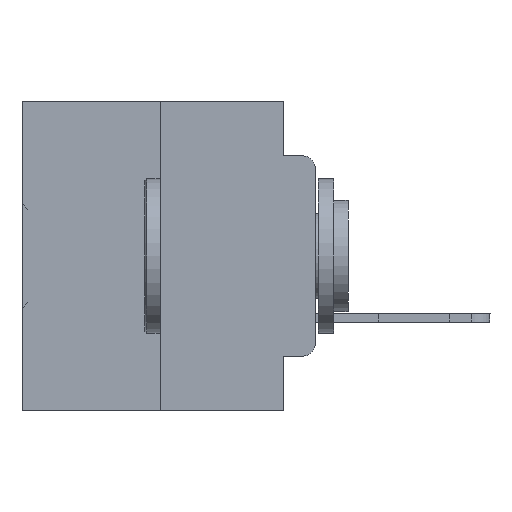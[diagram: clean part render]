
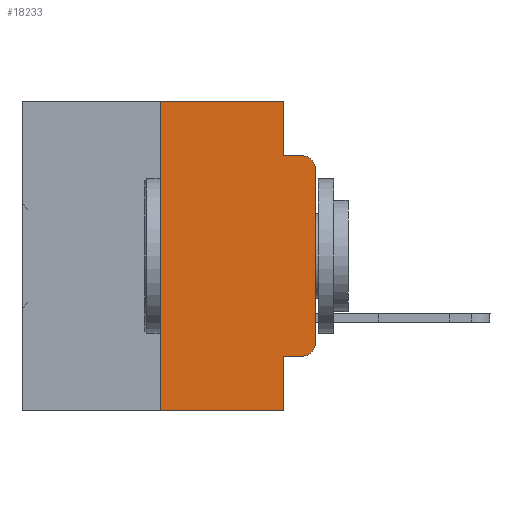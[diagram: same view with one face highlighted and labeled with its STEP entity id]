
A CAD part, left-side view. The second image highlights one B-rep face of the part: STEP entity #18233.
In plain terms, the highlighted planar face has unit normal (-1, 0, 0).
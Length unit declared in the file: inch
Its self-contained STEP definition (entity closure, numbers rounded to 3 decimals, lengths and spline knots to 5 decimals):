
#731 = VECTOR ( 'NONE', #1885, 39.37008 ) ;
#1237 = ORIENTED_EDGE ( 'NONE', *, *, #8486, .T. ) ;
#1719 = ORIENTED_EDGE ( 'NONE', *, *, #9011, .F. ) ;
#1763 = LINE ( 'NONE', #30060, #22072 ) ;
#1885 = DIRECTION ( 'NONE',  ( 0., 0., 1. ) ) ;
#2205 = CARTESIAN_POINT ( 'NONE',  ( 0., 0.051, -0.0885 ) ) ;
#2708 = EDGE_CURVE ( 'NONE', #35012, #25042, #12166, .T. ) ;
#3097 = VECTOR ( 'NONE', #13421, 39.37008 ) ;
#3600 = VERTEX_POINT ( 'NONE', #12506 ) ;
#4417 = VECTOR ( 'NONE', #28059, 39.37008 ) ;
#4917 = VERTEX_POINT ( 'NONE', #30510 ) ;
#5630 = EDGE_CURVE ( 'NONE', #26886, #35012, #10005, .T. ) ;
#7208 = CARTESIAN_POINT ( 'NONE',  ( 0., 0.051, 0. ) ) ;
#7951 = LINE ( 'NONE', #27059, #731 ) ;
#8177 = AXIS2_PLACEMENT_3D ( 'NONE', #26456, #20587, #17281 ) ;
#8486 = EDGE_CURVE ( 'NONE', #32466, #12380, #28861, .T. ) ;
#9011 = EDGE_CURVE ( 'NONE', #24558, #26886, #1763, .T. ) ;
#9212 = CARTESIAN_POINT ( 'NONE',  ( 0., 0.473, -0.5 ) ) ;
#9287 = ORIENTED_EDGE ( 'NONE', *, *, #27352, .T. ) ;
#10005 = LINE ( 'NONE', #26354, #25162 ) ;
#10825 = ORIENTED_EDGE ( 'NONE', *, *, #32022, .T. ) ;
#11792 = LINE ( 'NONE', #9212, #34590 ) ;
#11999 = CARTESIAN_POINT ( 'NONE',  ( 0., 0.051, -0.5 ) ) ;
#12124 = CARTESIAN_POINT ( 'NONE',  ( 0., 0.02, -0.0885 ) ) ;
#12166 = LINE ( 'NONE', #7208, #24839 ) ;
#12380 = VERTEX_POINT ( 'NONE', #19814 ) ;
#12393 = ORIENTED_EDGE ( 'NONE', *, *, #27799, .F. ) ;
#12506 = CARTESIAN_POINT ( 'NONE',  ( 0., 0., -0.1085 ) ) ;
#12562 = CARTESIAN_POINT ( 'NONE',  ( 0., 0.051, -0.0885 ) ) ;
#13025 = AXIS2_PLACEMENT_3D ( 'NONE', #31280, #15085, #17308 ) ;
#13421 = DIRECTION ( 'NONE',  ( 0., -1., 0. ) ) ;
#13905 = CARTESIAN_POINT ( 'NONE',  ( 0., 0.051, -0.4115 ) ) ;
#14605 = EDGE_CURVE ( 'NONE', #4917, #25969, #35206, .T. ) ;
#15085 = DIRECTION ( 'NONE',  ( -1., 0., 0. ) ) ;
#15254 = PLANE ( 'NONE',  #8177 ) ;
#16268 = DIRECTION ( 'NONE',  ( 0., 0., 1. ) ) ;
#17223 = ORIENTED_EDGE ( 'NONE', *, *, #20715, .T. ) ;
#17281 = DIRECTION ( 'NONE',  ( 0., 0., -1. ) ) ;
#17308 = DIRECTION ( 'NONE',  ( 0., 0., -1. ) ) ;
#17458 = FACE_OUTER_BOUND ( 'NONE', #34697, .T. ) ;
#18233 = ADVANCED_FACE ( 'NONE', ( #17458 ), #15254, .F. ) ;
#18416 = DIRECTION ( 'NONE',  ( 0., 0., -1. ) ) ;
#18717 = CARTESIAN_POINT ( 'NONE',  ( 0., 0.02, -0.1085 ) ) ;
#19814 = CARTESIAN_POINT ( 'NONE',  ( 0., 0., -0.3915 ) ) ;
#20587 = DIRECTION ( 'NONE',  ( 1., 0., 0. ) ) ;
#20715 = EDGE_CURVE ( 'NONE', #24558, #25969, #11792, .T. ) ;
#21419 = ORIENTED_EDGE ( 'NONE', *, *, #5630, .F. ) ;
#21574 = ORIENTED_EDGE ( 'NONE', *, *, #14605, .F. ) ;
#22072 = VECTOR ( 'NONE', #16268, 39.37008 ) ;
#22967 = VERTEX_POINT ( 'NONE', #12124 ) ;
#23923 = AXIS2_PLACEMENT_3D ( 'NONE', #18717, #35254, #29911 ) ;
#24558 = VERTEX_POINT ( 'NONE', #28635 ) ;
#24839 = VECTOR ( 'NONE', #18416, 39.37008 ) ;
#25042 = VERTEX_POINT ( 'NONE', #12562 ) ;
#25162 = VECTOR ( 'NONE', #34815, 39.37008 ) ;
#25969 = VERTEX_POINT ( 'NONE', #11999 ) ;
#26069 = ORIENTED_EDGE ( 'NONE', *, *, #2708, .F. ) ;
#26354 = CARTESIAN_POINT ( 'NONE',  ( 0., 0.473, 0. ) ) ;
#26383 = DIRECTION ( 'NONE',  ( 0., 0., -1. ) ) ;
#26456 = CARTESIAN_POINT ( 'NONE',  ( 0., 0.473, 0. ) ) ;
#26886 = VERTEX_POINT ( 'NONE', #32130 ) ;
#27059 = CARTESIAN_POINT ( 'NONE',  ( 0., 0., 0. ) ) ;
#27352 = EDGE_CURVE ( 'NONE', #12380, #3600, #7951, .T. ) ;
#27799 = EDGE_CURVE ( 'NONE', #25042, #22967, #32536, .T. ) ;
#28059 = DIRECTION ( 'NONE',  ( 0., -1., 0. ) ) ;
#28635 = CARTESIAN_POINT ( 'NONE',  ( 0., 0.25, -0.5 ) ) ;
#28861 = CIRCLE ( 'NONE', #13025, 0.02 ) ;
#29911 = DIRECTION ( 'NONE',  ( 0., 0., -1. ) ) ;
#30060 = CARTESIAN_POINT ( 'NONE',  ( 0., 0.25, 0. ) ) ;
#30087 = LINE ( 'NONE', #13905, #4417 ) ;
#30510 = CARTESIAN_POINT ( 'NONE',  ( 0., 0.051, -0.4115 ) ) ;
#31280 = CARTESIAN_POINT ( 'NONE',  ( 0., 0.02, -0.3915 ) ) ;
#31442 = DIRECTION ( 'NONE',  ( 0., -1., 0. ) ) ;
#31997 = CARTESIAN_POINT ( 'NONE',  ( 0., 0.051, 0. ) ) ;
#32022 = EDGE_CURVE ( 'NONE', #4917, #32466, #30087, .T. ) ;
#32130 = CARTESIAN_POINT ( 'NONE',  ( 0., 0.25, 0. ) ) ;
#32466 = VERTEX_POINT ( 'NONE', #35937 ) ;
#32536 = LINE ( 'NONE', #2205, #3097 ) ;
#33155 = ORIENTED_EDGE ( 'NONE', *, *, #34336, .T. ) ;
#34336 = EDGE_CURVE ( 'NONE', #3600, #22967, #36279, .T. ) ;
#34455 = VECTOR ( 'NONE', #26383, 39.37008 ) ;
#34590 = VECTOR ( 'NONE', #31442, 39.37008 ) ;
#34697 = EDGE_LOOP ( 'NONE', ( #9287, #33155, #12393, #26069, #21419, #1719, #17223, #21574, #10825, #1237 ) ) ;
#34815 = DIRECTION ( 'NONE',  ( 0., -1., 0. ) ) ;
#35012 = VERTEX_POINT ( 'NONE', #31997 ) ;
#35019 = CARTESIAN_POINT ( 'NONE',  ( 0., 0.051, 0. ) ) ;
#35206 = LINE ( 'NONE', #35019, #34455 ) ;
#35254 = DIRECTION ( 'NONE',  ( -1., 0., 0. ) ) ;
#35937 = CARTESIAN_POINT ( 'NONE',  ( 0., 0.02, -0.4115 ) ) ;
#36279 = CIRCLE ( 'NONE', #23923, 0.02 ) ;
